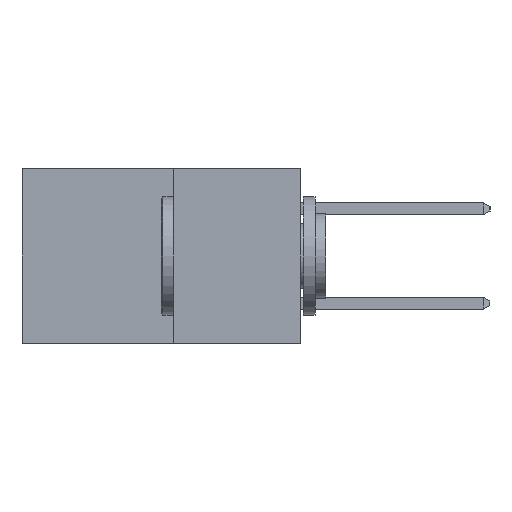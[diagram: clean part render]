
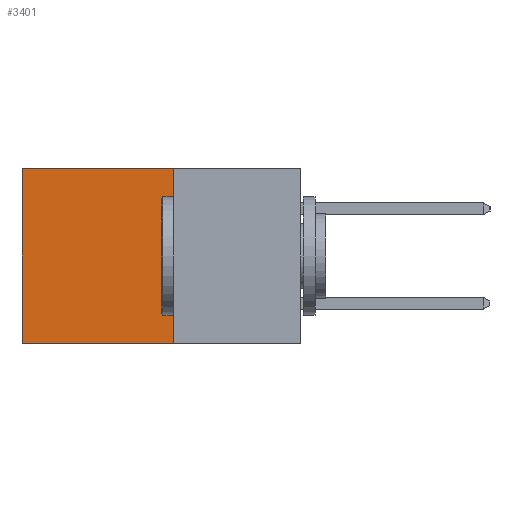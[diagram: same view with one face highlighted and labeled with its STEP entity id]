
A CAD part, left-side view. The second image highlights one B-rep face of the part: STEP entity #3401.
In plain terms, the highlighted planar face has unit normal (-1, 0, 0).
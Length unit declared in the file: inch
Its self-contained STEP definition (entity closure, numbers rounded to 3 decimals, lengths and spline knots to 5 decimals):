
#568 = LINE ( 'NONE', #2506, #10541 ) ;
#901 = VERTEX_POINT ( 'NONE', #4986 ) ;
#1068 = CARTESIAN_POINT ( 'NONE',  ( 0.277, 0.59, -0.37 ) ) ;
#1722 = FACE_OUTER_BOUND ( 'NONE', #10694, .T. ) ;
#2082 = EDGE_CURVE ( 'NONE', #4127, #901, #568, .T. ) ;
#2506 = CARTESIAN_POINT ( 'NONE',  ( 0.277, 0.27, 0. ) ) ;
#2639 = VERTEX_POINT ( 'NONE', #3921 ) ;
#3401 = ADVANCED_FACE ( 'NONE', ( #1722 ), #5129, .F. ) ;
#3921 = CARTESIAN_POINT ( 'NONE',  ( 0.277, 0.59, -0.37 ) ) ;
#4127 = VERTEX_POINT ( 'NONE', #5746 ) ;
#4899 = VERTEX_POINT ( 'NONE', #11852 ) ;
#4986 = CARTESIAN_POINT ( 'NONE',  ( 0.277, 0.59, 0. ) ) ;
#5083 = EDGE_CURVE ( 'NONE', #4899, #2639, #9243, .T. ) ;
#5129 = PLANE ( 'NONE',  #9354 ) ;
#5144 = DIRECTION ( 'NONE',  ( 1., 0., 0. ) ) ;
#5338 = DIRECTION ( 'NONE',  ( 0., 0., -1. ) ) ;
#5746 = CARTESIAN_POINT ( 'NONE',  ( 0.277, 0.27, 0. ) ) ;
#5799 = DIRECTION ( 'NONE',  ( 0., 0., -1. ) ) ;
#6063 = CARTESIAN_POINT ( 'NONE',  ( 0.277, 0.27, -0.37 ) ) ;
#6141 = VECTOR ( 'NONE', #7270, 39.37008 ) ;
#6260 = ORIENTED_EDGE ( 'NONE', *, *, #8390, .T. ) ;
#6330 = ORIENTED_EDGE ( 'NONE', *, *, #5083, .F. ) ;
#6343 = ORIENTED_EDGE ( 'NONE', *, *, #9289, .F. ) ;
#6432 = ORIENTED_EDGE ( 'NONE', *, *, #2082, .T. ) ;
#7270 = DIRECTION ( 'NONE',  ( 0., 1., 0. ) ) ;
#7291 = VECTOR ( 'NONE', #5799, 39.37008 ) ;
#7380 = CARTESIAN_POINT ( 'NONE',  ( 0.277, 0.27, -0.37 ) ) ;
#7679 = DIRECTION ( 'NONE',  ( 0., 0., -1. ) ) ;
#8120 = DIRECTION ( 'NONE',  ( 0., 1., 0. ) ) ;
#8390 = EDGE_CURVE ( 'NONE', #901, #2639, #8664, .T. ) ;
#8664 = LINE ( 'NONE', #1068, #8951 ) ;
#8951 = VECTOR ( 'NONE', #7679, 39.37008 ) ;
#9243 = LINE ( 'NONE', #7380, #6141 ) ;
#9289 = EDGE_CURVE ( 'NONE', #4127, #4899, #9764, .T. ) ;
#9354 = AXIS2_PLACEMENT_3D ( 'NONE', #6063, #5144, #5338 ) ;
#9533 = CARTESIAN_POINT ( 'NONE',  ( 0.277, 0.27, -0.37 ) ) ;
#9764 = LINE ( 'NONE', #9533, #7291 ) ;
#10541 = VECTOR ( 'NONE', #8120, 39.37008 ) ;
#10694 = EDGE_LOOP ( 'NONE', ( #6260, #6330, #6343, #6432 ) ) ;
#11852 = CARTESIAN_POINT ( 'NONE',  ( 0.277, 0.27, -0.37 ) ) ;
